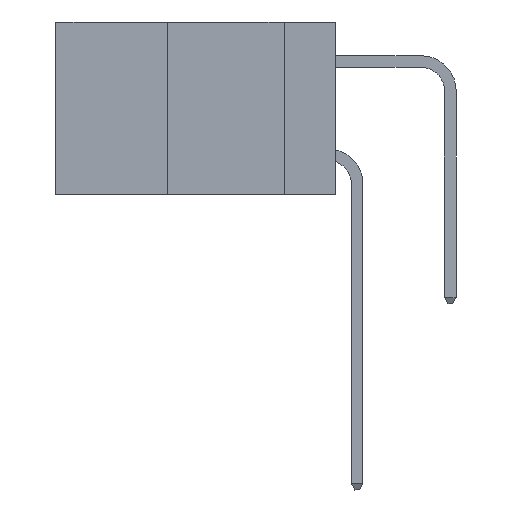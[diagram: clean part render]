
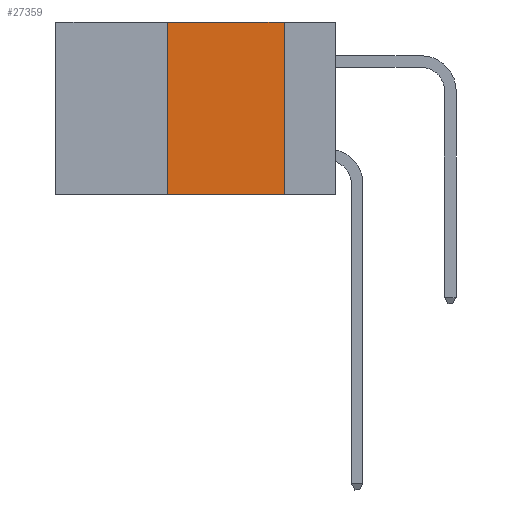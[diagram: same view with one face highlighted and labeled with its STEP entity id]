
A CAD part, left-side view. The second image highlights one B-rep face of the part: STEP entity #27359.
In plain terms, the highlighted planar face has unit normal (-1, 0, 0).
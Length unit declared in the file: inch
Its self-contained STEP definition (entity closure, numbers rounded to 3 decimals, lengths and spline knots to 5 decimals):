
#401 = VECTOR ( 'NONE', #31061, 39.37008 ) ;
#2478 = FACE_OUTER_BOUND ( 'NONE', #42254, .T. ) ;
#2695 = ORIENTED_EDGE ( 'NONE', *, *, #22103, .T. ) ;
#6201 = CARTESIAN_POINT ( 'NONE',  ( 0., 0.6, 0. ) ) ;
#7651 = DIRECTION ( 'NONE',  ( 0., 0., 1. ) ) ;
#8088 = CARTESIAN_POINT ( 'NONE',  ( 0., 0.11, 0. ) ) ;
#8499 = LINE ( 'NONE', #32059, #25049 ) ;
#10849 = VERTEX_POINT ( 'NONE', #31099 ) ;
#12756 = CARTESIAN_POINT ( 'NONE',  ( 0., 0.11, 0. ) ) ;
#13099 = VERTEX_POINT ( 'NONE', #8088 ) ;
#13359 = VERTEX_POINT ( 'NONE', #23943 ) ;
#16414 = DIRECTION ( 'NONE',  ( 0., 0., -1. ) ) ;
#16633 = ORIENTED_EDGE ( 'NONE', *, *, #37184, .F. ) ;
#18425 = VECTOR ( 'NONE', #41776, 39.37008 ) ;
#20402 = PLANE ( 'NONE',  #40719 ) ;
#22103 = EDGE_CURVE ( 'NONE', #13359, #29395, #25070, .T. ) ;
#23943 = CARTESIAN_POINT ( 'NONE',  ( 0., 0.36, -0.37 ) ) ;
#23964 = DIRECTION ( 'NONE',  ( 1., 0., 0. ) ) ;
#24410 = EDGE_CURVE ( 'NONE', #13099, #29395, #43597, .T. ) ;
#25049 = VECTOR ( 'NONE', #7651, 39.37008 ) ;
#25070 = LINE ( 'NONE', #30714, #18425 ) ;
#26415 = LINE ( 'NONE', #34596, #401 ) ;
#27359 = ADVANCED_FACE ( 'NONE', ( #2478 ), #20402, .F. ) ;
#29395 = VERTEX_POINT ( 'NONE', #38931 ) ;
#30714 = CARTESIAN_POINT ( 'NONE',  ( 0., 0.6, -0.37 ) ) ;
#31061 = DIRECTION ( 'NONE',  ( 0., -1., 0. ) ) ;
#31099 = CARTESIAN_POINT ( 'NONE',  ( 0., 0.36, 0. ) ) ;
#32059 = CARTESIAN_POINT ( 'NONE',  ( 0., 0.36, 0. ) ) ;
#34596 = CARTESIAN_POINT ( 'NONE',  ( 0., 0.6, 0. ) ) ;
#37184 = EDGE_CURVE ( 'NONE', #13359, #10849, #8499, .T. ) ;
#37239 = ORIENTED_EDGE ( 'NONE', *, *, #24410, .F. ) ;
#37549 = VECTOR ( 'NONE', #40371, 39.37008 ) ;
#38931 = CARTESIAN_POINT ( 'NONE',  ( 0., 0.11, -0.37 ) ) ;
#40371 = DIRECTION ( 'NONE',  ( 0., 0., -1. ) ) ;
#40582 = EDGE_CURVE ( 'NONE', #10849, #13099, #26415, .T. ) ;
#40719 = AXIS2_PLACEMENT_3D ( 'NONE', #6201, #23964, #16414 ) ;
#41776 = DIRECTION ( 'NONE',  ( 0., -1., 0. ) ) ;
#42254 = EDGE_LOOP ( 'NONE', ( #37239, #43067, #16633, #2695 ) ) ;
#43067 = ORIENTED_EDGE ( 'NONE', *, *, #40582, .F. ) ;
#43597 = LINE ( 'NONE', #12756, #37549 ) ;
